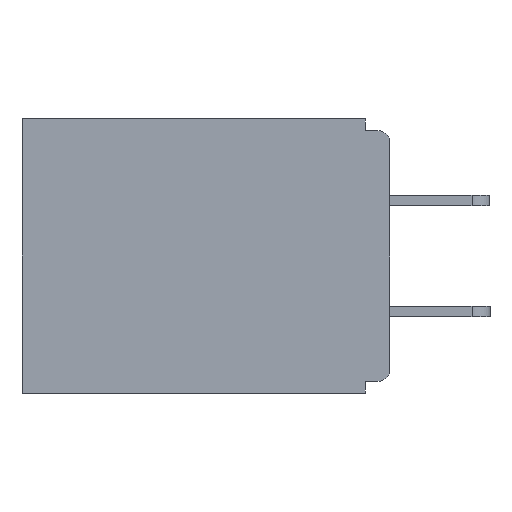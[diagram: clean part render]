
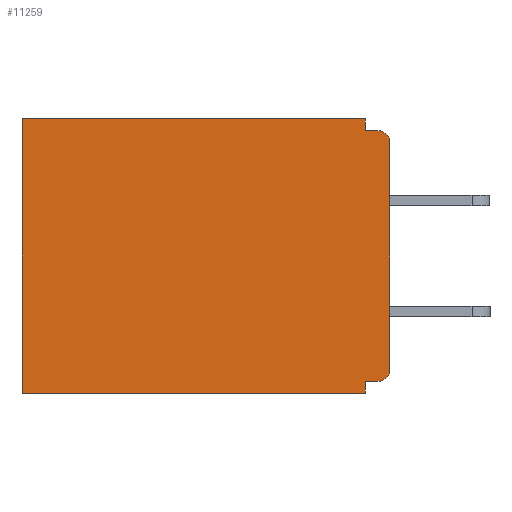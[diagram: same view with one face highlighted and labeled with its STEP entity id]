
A CAD part, left-side view. The second image highlights one B-rep face of the part: STEP entity #11259.
In plain terms, the highlighted planar face has unit normal (-1, 0, 0).
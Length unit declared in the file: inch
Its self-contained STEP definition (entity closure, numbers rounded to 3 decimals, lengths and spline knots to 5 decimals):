
#221 = LINE ( 'NONE', #11422, #8435 ) ;
#506 = CARTESIAN_POINT ( 'NONE',  ( 0.298, 0., 0. ) ) ;
#555 = EDGE_CURVE ( 'NONE', #5641, #11648, #9564, .T. ) ;
#666 = CARTESIAN_POINT ( 'NONE',  ( 0.298, 0., -0.343 ) ) ;
#905 = CARTESIAN_POINT ( 'NONE',  ( 0.298, 0., -0.03 ) ) ;
#1039 = VERTEX_POINT ( 'NONE', #6467 ) ;
#1423 = CARTESIAN_POINT ( 'NONE',  ( 0.298, 0.031, -0.328 ) ) ;
#1744 = AXIS2_PLACEMENT_3D ( 'NONE', #5149, #7265, #5107 ) ;
#1881 = CARTESIAN_POINT ( 'NONE',  ( 0.298, 0., -0.328 ) ) ;
#2023 = ORIENTED_EDGE ( 'NONE', *, *, #6434, .F. ) ;
#2064 = ORIENTED_EDGE ( 'NONE', *, *, #10846, .F. ) ;
#2275 = VERTEX_POINT ( 'NONE', #8366 ) ;
#2298 = CARTESIAN_POINT ( 'NONE',  ( 0.298, 0.031, -0.343 ) ) ;
#2328 = ORIENTED_EDGE ( 'NONE', *, *, #9839, .T. ) ;
#2388 = DIRECTION ( 'NONE',  ( 0., 0., -1. ) ) ;
#2704 = DIRECTION ( 'NONE',  ( 0., 0., -1. ) ) ;
#2741 = ORIENTED_EDGE ( 'NONE', *, *, #12900, .F. ) ;
#2785 = DIRECTION ( 'NONE',  ( 0., 1., 0. ) ) ;
#3033 = DIRECTION ( 'NONE',  ( 0., 0., -1. ) ) ;
#3069 = CARTESIAN_POINT ( 'NONE',  ( 0.298, 0.031, -0.015 ) ) ;
#3188 = AXIS2_PLACEMENT_3D ( 'NONE', #7774, #8774, #2704 ) ;
#3345 = PLANE ( 'NONE',  #12000 ) ;
#3666 = VECTOR ( 'NONE', #2388, 39.37008 ) ;
#3747 = EDGE_CURVE ( 'NONE', #5641, #12695, #12312, .T. ) ;
#3983 = CARTESIAN_POINT ( 'NONE',  ( 0.298, 0.031, -0.343 ) ) ;
#4412 = CARTESIAN_POINT ( 'NONE',  ( 0.298, 0., 0. ) ) ;
#4424 = CARTESIAN_POINT ( 'NONE',  ( 0.298, 0.031, 0. ) ) ;
#4648 = FACE_OUTER_BOUND ( 'NONE', #8574, .T. ) ;
#4660 = EDGE_CURVE ( 'NONE', #9688, #1039, #7416, .T. ) ;
#5107 = DIRECTION ( 'NONE',  ( 0., 0., -1. ) ) ;
#5149 = CARTESIAN_POINT ( 'NONE',  ( 0.298, 0.015, -0.03 ) ) ;
#5330 = CIRCLE ( 'NONE', #3188, 0.015 ) ;
#5411 = CARTESIAN_POINT ( 'NONE',  ( 0.298, 0.46, 0. ) ) ;
#5432 = DIRECTION ( 'NONE',  ( 0., 0., -1. ) ) ;
#5538 = CARTESIAN_POINT ( 'NONE',  ( 0.298, 0., -0.313 ) ) ;
#5623 = CARTESIAN_POINT ( 'NONE',  ( 0.298, 0.46, -0.343 ) ) ;
#5630 = DIRECTION ( 'NONE',  ( 0., 1., 0. ) ) ;
#5641 = VERTEX_POINT ( 'NONE', #4424 ) ;
#6434 = EDGE_CURVE ( 'NONE', #9688, #8357, #12057, .T. ) ;
#6467 = CARTESIAN_POINT ( 'NONE',  ( 0.298, 0.015, -0.015 ) ) ;
#6971 = CARTESIAN_POINT ( 'NONE',  ( 0.298, 0.46, 0. ) ) ;
#7154 = ORIENTED_EDGE ( 'NONE', *, *, #8666, .T. ) ;
#7265 = DIRECTION ( 'NONE',  ( -1., 0., 0. ) ) ;
#7416 = CIRCLE ( 'NONE', #1744, 0.015 ) ;
#7448 = LINE ( 'NONE', #5411, #12798 ) ;
#7511 = VERTEX_POINT ( 'NONE', #1423 ) ;
#7766 = DIRECTION ( 'NONE',  ( 0., 1., 0. ) ) ;
#7774 = CARTESIAN_POINT ( 'NONE',  ( 0.298, 0.015, -0.313 ) ) ;
#8196 = ORIENTED_EDGE ( 'NONE', *, *, #3747, .T. ) ;
#8284 = VECTOR ( 'NONE', #5630, 39.37008 ) ;
#8357 = VERTEX_POINT ( 'NONE', #5538 ) ;
#8366 = CARTESIAN_POINT ( 'NONE',  ( 0.298, 0.031, -0.343 ) ) ;
#8435 = VECTOR ( 'NONE', #11515, 39.37008 ) ;
#8574 = EDGE_LOOP ( 'NONE', ( #9004, #10762, #11835, #8196, #7154, #2741, #9071, #2064, #2328, #2023 ) ) ;
#8666 = EDGE_CURVE ( 'NONE', #12695, #11966, #7448, .T. ) ;
#8739 = VECTOR ( 'NONE', #7766, 39.37008 ) ;
#8774 = DIRECTION ( 'NONE',  ( -1., 0., 0. ) ) ;
#8792 = DIRECTION ( 'NONE',  ( 0., 0., -1. ) ) ;
#9004 = ORIENTED_EDGE ( 'NONE', *, *, #4660, .T. ) ;
#9071 = ORIENTED_EDGE ( 'NONE', *, *, #12485, .F. ) ;
#9117 = LINE ( 'NONE', #2298, #3666 ) ;
#9564 = LINE ( 'NONE', #3983, #12853 ) ;
#9688 = VERTEX_POINT ( 'NONE', #905 ) ;
#9839 = EDGE_CURVE ( 'NONE', #13305, #8357, #5330, .T. ) ;
#10409 = CARTESIAN_POINT ( 'NONE',  ( 0.298, 0.015, -0.328 ) ) ;
#10762 = ORIENTED_EDGE ( 'NONE', *, *, #13234, .F. ) ;
#10787 = LINE ( 'NONE', #1881, #11439 ) ;
#10846 = EDGE_CURVE ( 'NONE', #13305, #7511, #10787, .T. ) ;
#11259 = ADVANCED_FACE ( 'NONE', ( #4648 ), #3345, .F. ) ;
#11377 = LINE ( 'NONE', #666, #8284 ) ;
#11422 = CARTESIAN_POINT ( 'NONE',  ( 0.298, 0., -0.015 ) ) ;
#11425 = DIRECTION ( 'NONE',  ( 1., 0., 0. ) ) ;
#11439 = VECTOR ( 'NONE', #2785, 39.37008 ) ;
#11496 = DIRECTION ( 'NONE',  ( 0., 0., -1. ) ) ;
#11515 = DIRECTION ( 'NONE',  ( 0., -1., 0. ) ) ;
#11648 = VERTEX_POINT ( 'NONE', #3069 ) ;
#11835 = ORIENTED_EDGE ( 'NONE', *, *, #555, .F. ) ;
#11966 = VERTEX_POINT ( 'NONE', #5623 ) ;
#12000 = AXIS2_PLACEMENT_3D ( 'NONE', #4412, #11425, #5432 ) ;
#12057 = LINE ( 'NONE', #506, #12373 ) ;
#12312 = LINE ( 'NONE', #13165, #8739 ) ;
#12373 = VECTOR ( 'NONE', #8792, 39.37008 ) ;
#12485 = EDGE_CURVE ( 'NONE', #7511, #2275, #9117, .T. ) ;
#12695 = VERTEX_POINT ( 'NONE', #6971 ) ;
#12798 = VECTOR ( 'NONE', #11496, 39.37008 ) ;
#12853 = VECTOR ( 'NONE', #3033, 39.37008 ) ;
#12900 = EDGE_CURVE ( 'NONE', #2275, #11966, #11377, .T. ) ;
#13165 = CARTESIAN_POINT ( 'NONE',  ( 0.298, 0., 0. ) ) ;
#13234 = EDGE_CURVE ( 'NONE', #11648, #1039, #221, .T. ) ;
#13305 = VERTEX_POINT ( 'NONE', #10409 ) ;
